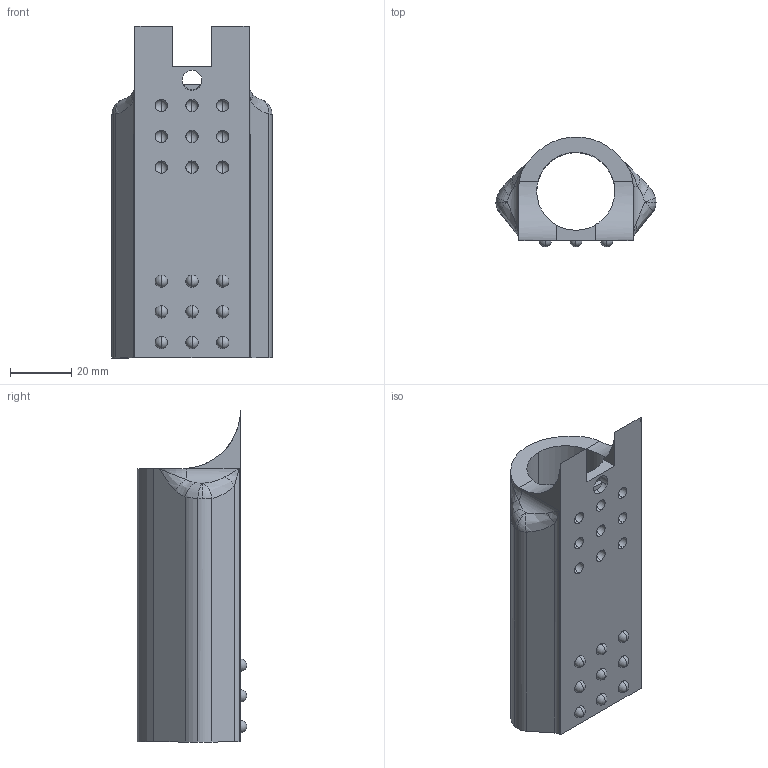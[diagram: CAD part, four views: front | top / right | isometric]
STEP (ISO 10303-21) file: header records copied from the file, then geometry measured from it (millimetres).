
FILE_DESCRIPTION (( 'STEP AP214' ), '1' );
FILE_NAME ('Buffer_Tube_1b.STEP', '2013-09-01T16:38:34', ( 'Asher' ), ( '' ), 'SwSTEP 2.0', 'SolidWorks 2013', '' );
FILE_SCHEMA (( 'AUTOMOTIVE_DESIGN' ));
Length unit declared in the file: millimetre
Products named in the file (1): Buffer_Tube_1b
Bounding box: 52.09 x 35.59 x 108 mm (x, y, z)
Volume: 72336.9 mm3; surface area: 22133.8 mm2
Topology: 1 solids, 1 shells, 86 faces, 273 edges, 165 vertices
Faces by surface type: sphere 40, cylinder 18, plane 14, bspline 12, torus 2
Entity records: 3004 total; most frequent: CARTESIAN_POINT 1025, DIRECTION 427, ORIENTED_EDGE 394, EDGE_CURVE 197, AXIS2_PLACEMENT_3D 190, VERTEX_POINT 129, CIRCLE 115, EDGE_LOOP 106
